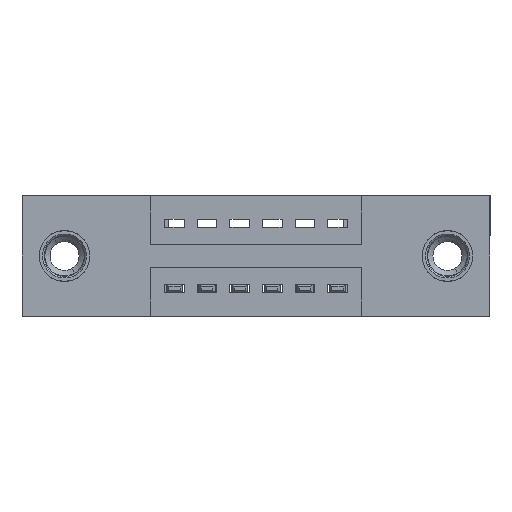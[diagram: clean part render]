
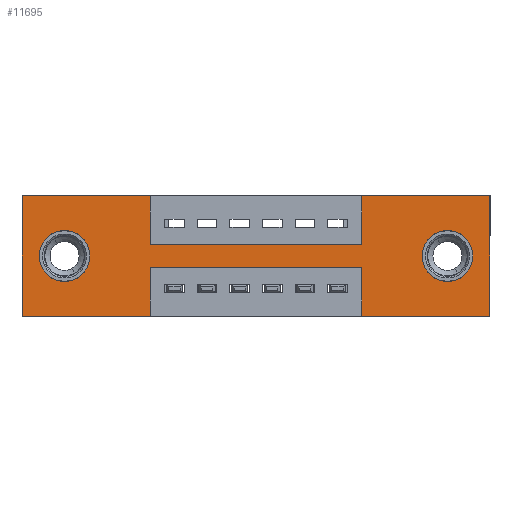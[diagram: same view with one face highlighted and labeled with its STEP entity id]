
A CAD part, front view. The second image highlights one B-rep face of the part: STEP entity #11695.
In plain terms, the highlighted planar face has unit normal (0, -1, 0).
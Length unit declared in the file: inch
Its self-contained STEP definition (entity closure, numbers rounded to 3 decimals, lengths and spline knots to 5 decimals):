
#152 = ORIENTED_EDGE ( 'NONE', *, *, #8817, .F. ) ;
#229 = EDGE_CURVE ( 'NONE', #4878, #2867, #13143, .T. ) ;
#241 = LINE ( 'NONE', #2565, #1752 ) ;
#420 = EDGE_LOOP ( 'NONE', ( #152, #2226, #10198, #7458, #10374, #5704, #4394, #11488, #7642, #2351, #12357, #8898 ) ) ;
#519 = VERTEX_POINT ( 'NONE', #11130 ) ;
#557 = CARTESIAN_POINT ( 'NONE',  ( 1.435, 0., -0.37 ) ) ;
#1048 = CARTESIAN_POINT ( 'NONE',  ( 0.13, 0., -0.185 ) ) ;
#1086 = AXIS2_PLACEMENT_3D ( 'NONE', #1048, #11821, #10860 ) ;
#1228 = CARTESIAN_POINT ( 'NONE',  ( 0., 0., -0.37 ) ) ;
#1261 = VECTOR ( 'NONE', #6589, 39.37008 ) ;
#1281 = CARTESIAN_POINT ( 'NONE',  ( 0.3925, 0., 0. ) ) ;
#1346 = DIRECTION ( 'NONE',  ( 1., 0., 0. ) ) ;
#1489 = DIRECTION ( 'NONE',  ( -1., 0., 0. ) ) ;
#1556 = CARTESIAN_POINT ( 'NONE',  ( 0.13, 0., -0.107 ) ) ;
#1724 = ORIENTED_EDGE ( 'NONE', *, *, #7172, .T. ) ;
#1741 = DIRECTION ( 'NONE',  ( 0., 0., -1. ) ) ;
#1752 = VECTOR ( 'NONE', #3086, 39.37008 ) ;
#1933 = VERTEX_POINT ( 'NONE', #1974 ) ;
#1974 = CARTESIAN_POINT ( 'NONE',  ( 1.0425, 0., -0.22 ) ) ;
#2190 = VECTOR ( 'NONE', #6257, 39.37008 ) ;
#2226 = ORIENTED_EDGE ( 'NONE', *, *, #9913, .F. ) ;
#2246 = CIRCLE ( 'NONE', #1086, 0.078 ) ;
#2351 = ORIENTED_EDGE ( 'NONE', *, *, #3951, .F. ) ;
#2445 = CARTESIAN_POINT ( 'NONE',  ( 0.3925, 0., -0.15 ) ) ;
#2565 = CARTESIAN_POINT ( 'NONE',  ( 0.3925, 0., -0.22 ) ) ;
#2622 = DIRECTION ( 'NONE',  ( 0., 0., 1. ) ) ;
#2867 = VERTEX_POINT ( 'NONE', #8452 ) ;
#2992 = CARTESIAN_POINT ( 'NONE',  ( 1.305, 0., -0.185 ) ) ;
#3086 = DIRECTION ( 'NONE',  ( -1., 0., 0. ) ) ;
#3104 = DIRECTION ( 'NONE',  ( 0., 0., 1. ) ) ;
#3311 = CARTESIAN_POINT ( 'NONE',  ( 0.3925, 0., -0.22 ) ) ;
#3439 = CARTESIAN_POINT ( 'NONE',  ( 0.3925, 0., -0.37 ) ) ;
#3448 = VERTEX_POINT ( 'NONE', #10246 ) ;
#3867 = PLANE ( 'NONE',  #5724 ) ;
#3951 = EDGE_CURVE ( 'NONE', #4693, #5460, #8305, .T. ) ;
#3994 = DIRECTION ( 'NONE',  ( 0., -1., 0. ) ) ;
#4075 = EDGE_CURVE ( 'NONE', #7395, #7760, #13182, .T. ) ;
#4138 = LINE ( 'NONE', #3439, #1261 ) ;
#4263 = EDGE_CURVE ( 'NONE', #2867, #8975, #10166, .T. ) ;
#4394 = ORIENTED_EDGE ( 'NONE', *, *, #4263, .F. ) ;
#4474 = VERTEX_POINT ( 'NONE', #13044 ) ;
#4490 = CARTESIAN_POINT ( 'NONE',  ( 0.13, 0., -0.185 ) ) ;
#4538 = EDGE_LOOP ( 'NONE', ( #8482, #7652 ) ) ;
#4601 = DIRECTION ( 'NONE',  ( 0., 0., -1. ) ) ;
#4603 = VECTOR ( 'NONE', #11028, 39.37008 ) ;
#4693 = VERTEX_POINT ( 'NONE', #10553 ) ;
#4694 = CARTESIAN_POINT ( 'NONE',  ( 1.0425, 0., -0.37 ) ) ;
#4793 = DIRECTION ( 'NONE',  ( 0., 0., 1. ) ) ;
#4878 = VERTEX_POINT ( 'NONE', #2445 ) ;
#5066 = VERTEX_POINT ( 'NONE', #1556 ) ;
#5152 = CARTESIAN_POINT ( 'NONE',  ( 1.305, 0., -0.263 ) ) ;
#5460 = VERTEX_POINT ( 'NONE', #1281 ) ;
#5545 = VERTEX_POINT ( 'NONE', #3311 ) ;
#5570 = FACE_OUTER_BOUND ( 'NONE', #420, .T. ) ;
#5644 = EDGE_LOOP ( 'NONE', ( #7379, #1724 ) ) ;
#5704 = ORIENTED_EDGE ( 'NONE', *, *, #9285, .F. ) ;
#5724 = AXIS2_PLACEMENT_3D ( 'NONE', #6239, #3994, #13764 ) ;
#5820 = VECTOR ( 'NONE', #1346, 39.37008 ) ;
#6201 = LINE ( 'NONE', #11529, #7726 ) ;
#6239 = CARTESIAN_POINT ( 'NONE',  ( 0., 0., -0.37 ) ) ;
#6257 = DIRECTION ( 'NONE',  ( 1., 0., 0. ) ) ;
#6346 = AXIS2_PLACEMENT_3D ( 'NONE', #2992, #10679, #10639 ) ;
#6362 = VERTEX_POINT ( 'NONE', #5152 ) ;
#6369 = VECTOR ( 'NONE', #7934, 39.37008 ) ;
#6541 = LINE ( 'NONE', #13877, #6369 ) ;
#6589 = DIRECTION ( 'NONE',  ( 0., 0., -1. ) ) ;
#6594 = VERTEX_POINT ( 'NONE', #12002 ) ;
#6749 = CARTESIAN_POINT ( 'NONE',  ( 1.305, 0., -0.185 ) ) ;
#6880 = EDGE_CURVE ( 'NONE', #7760, #4693, #6201, .T. ) ;
#7172 = EDGE_CURVE ( 'NONE', #6594, #5066, #13283, .T. ) ;
#7379 = ORIENTED_EDGE ( 'NONE', *, *, #10000, .T. ) ;
#7395 = VERTEX_POINT ( 'NONE', #9397 ) ;
#7415 = VECTOR ( 'NONE', #1741, 39.37008 ) ;
#7444 = LINE ( 'NONE', #13179, #4603 ) ;
#7458 = ORIENTED_EDGE ( 'NONE', *, *, #11075, .F. ) ;
#7480 = EDGE_CURVE ( 'NONE', #3448, #1933, #8741, .T. ) ;
#7642 = ORIENTED_EDGE ( 'NONE', *, *, #12150, .F. ) ;
#7652 = ORIENTED_EDGE ( 'NONE', *, *, #8626, .T. ) ;
#7662 = CARTESIAN_POINT ( 'NONE',  ( 1.0425, 0., 0. ) ) ;
#7726 = VECTOR ( 'NONE', #3104, 39.37008 ) ;
#7760 = VERTEX_POINT ( 'NONE', #1228 ) ;
#7786 = CARTESIAN_POINT ( 'NONE',  ( 0.3925, 0., 0. ) ) ;
#7934 = DIRECTION ( 'NONE',  ( 0., 0., -1. ) ) ;
#7991 = VECTOR ( 'NONE', #9009, 39.37008 ) ;
#8117 = LINE ( 'NONE', #7786, #7415 ) ;
#8293 = VECTOR ( 'NONE', #4793, 39.37008 ) ;
#8305 = LINE ( 'NONE', #12310, #7991 ) ;
#8429 = FACE_BOUND ( 'NONE', #5644, .T. ) ;
#8452 = CARTESIAN_POINT ( 'NONE',  ( 1.0425, 0., -0.15 ) ) ;
#8482 = ORIENTED_EDGE ( 'NONE', *, *, #12789, .T. ) ;
#8626 = EDGE_CURVE ( 'NONE', #6362, #519, #10247, .T. ) ;
#8741 = LINE ( 'NONE', #4694, #10592 ) ;
#8817 = EDGE_CURVE ( 'NONE', #5545, #7395, #4138, .T. ) ;
#8898 = ORIENTED_EDGE ( 'NONE', *, *, #4075, .F. ) ;
#8967 = DIRECTION ( 'NONE',  ( 0., 1., 0. ) ) ;
#8975 = VERTEX_POINT ( 'NONE', #7662 ) ;
#9009 = DIRECTION ( 'NONE',  ( 1., 0., 0. ) ) ;
#9285 = EDGE_CURVE ( 'NONE', #8975, #4474, #13410, .T. ) ;
#9397 = CARTESIAN_POINT ( 'NONE',  ( 0.3925, 0., -0.37 ) ) ;
#9399 = AXIS2_PLACEMENT_3D ( 'NONE', #6749, #10066, #4601 ) ;
#9443 = VERTEX_POINT ( 'NONE', #557 ) ;
#9861 = DIRECTION ( 'NONE',  ( 0., 0., 1. ) ) ;
#9913 = EDGE_CURVE ( 'NONE', #1933, #5545, #241, .T. ) ;
#9930 = CIRCLE ( 'NONE', #6346, 0.078 ) ;
#10000 = EDGE_CURVE ( 'NONE', #5066, #6594, #2246, .T. ) ;
#10066 = DIRECTION ( 'NONE',  ( 0., 1., 0. ) ) ;
#10166 = LINE ( 'NONE', #12341, #8293 ) ;
#10198 = ORIENTED_EDGE ( 'NONE', *, *, #7480, .F. ) ;
#10246 = CARTESIAN_POINT ( 'NONE',  ( 1.0425, 0., -0.37 ) ) ;
#10247 = CIRCLE ( 'NONE', #9399, 0.078 ) ;
#10340 = VECTOR ( 'NONE', #1489, 39.37008 ) ;
#10374 = ORIENTED_EDGE ( 'NONE', *, *, #13336, .F. ) ;
#10553 = CARTESIAN_POINT ( 'NONE',  ( 0., 0., 0. ) ) ;
#10592 = VECTOR ( 'NONE', #2622, 39.37008 ) ;
#10605 = CARTESIAN_POINT ( 'NONE',  ( 0.3925, 0., -0.15 ) ) ;
#10639 = DIRECTION ( 'NONE',  ( 0., 0., -1. ) ) ;
#10679 = DIRECTION ( 'NONE',  ( 0., 1., 0. ) ) ;
#10860 = DIRECTION ( 'NONE',  ( 0., 0., 1. ) ) ;
#11010 = CARTESIAN_POINT ( 'NONE',  ( 0., 0., -0.37 ) ) ;
#11028 = DIRECTION ( 'NONE',  ( -1., 0., 0. ) ) ;
#11075 = EDGE_CURVE ( 'NONE', #9443, #3448, #7444, .T. ) ;
#11130 = CARTESIAN_POINT ( 'NONE',  ( 1.305, 0., -0.107 ) ) ;
#11161 = FACE_BOUND ( 'NONE', #4538, .T. ) ;
#11488 = ORIENTED_EDGE ( 'NONE', *, *, #229, .F. ) ;
#11529 = CARTESIAN_POINT ( 'NONE',  ( 0., 0., 0. ) ) ;
#11695 = ADVANCED_FACE ( 'NONE', ( #11161, #8429, #5570 ), #3867, .T. ) ;
#11821 = DIRECTION ( 'NONE',  ( 0., 1., 0. ) ) ;
#12002 = CARTESIAN_POINT ( 'NONE',  ( 0.13, 0., -0.263 ) ) ;
#12150 = EDGE_CURVE ( 'NONE', #5460, #4878, #8117, .T. ) ;
#12164 = CARTESIAN_POINT ( 'NONE',  ( 0., 0., 0. ) ) ;
#12310 = CARTESIAN_POINT ( 'NONE',  ( 0., 0., 0. ) ) ;
#12341 = CARTESIAN_POINT ( 'NONE',  ( 1.0425, 0., 0. ) ) ;
#12357 = ORIENTED_EDGE ( 'NONE', *, *, #6880, .F. ) ;
#12789 = EDGE_CURVE ( 'NONE', #519, #6362, #9930, .T. ) ;
#13044 = CARTESIAN_POINT ( 'NONE',  ( 1.435, 0., 0. ) ) ;
#13143 = LINE ( 'NONE', #10605, #2190 ) ;
#13179 = CARTESIAN_POINT ( 'NONE',  ( 0., 0., -0.37 ) ) ;
#13182 = LINE ( 'NONE', #11010, #10340 ) ;
#13283 = CIRCLE ( 'NONE', #13620, 0.078 ) ;
#13336 = EDGE_CURVE ( 'NONE', #4474, #9443, #6541, .T. ) ;
#13410 = LINE ( 'NONE', #12164, #5820 ) ;
#13620 = AXIS2_PLACEMENT_3D ( 'NONE', #4490, #8967, #9861 ) ;
#13764 = DIRECTION ( 'NONE',  ( 0., 0., -1. ) ) ;
#13877 = CARTESIAN_POINT ( 'NONE',  ( 1.435, 0., 0. ) ) ;
